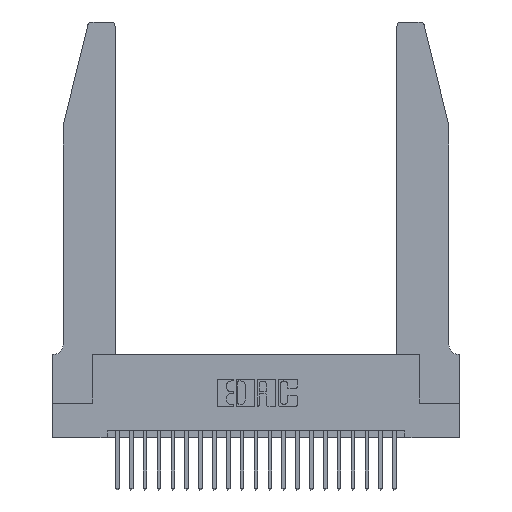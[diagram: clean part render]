
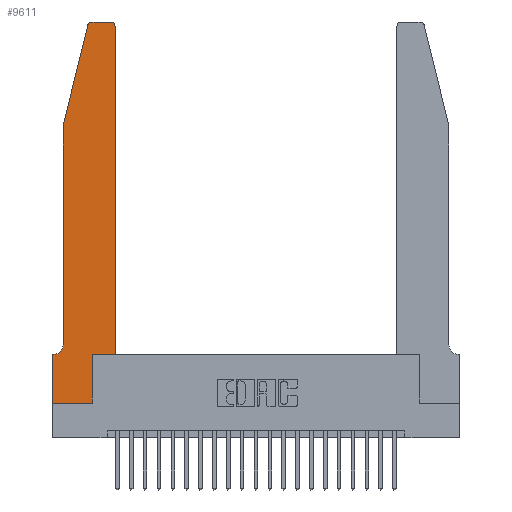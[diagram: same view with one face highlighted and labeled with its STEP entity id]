
A CAD part, top view. The second image highlights one B-rep face of the part: STEP entity #9611.
In plain terms, the highlighted planar face has unit normal (0, 0, 1).
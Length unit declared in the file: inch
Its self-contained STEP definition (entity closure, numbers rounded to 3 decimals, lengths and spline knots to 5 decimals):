
#337 = LINE ( 'NONE', #6783, #23899 ) ;
#454 = CARTESIAN_POINT ( 'NONE',  ( 0.4205, 2.75, 0.37 ) ) ;
#573 = CARTESIAN_POINT ( 'NONE',  ( 0.0055, 0.35, 0.37 ) ) ;
#661 = CARTESIAN_POINT ( 'NONE',  ( 0.284, 2.72, 0.37 ) ) ;
#675 = LINE ( 'NONE', #11678, #16179 ) ;
#829 = EDGE_CURVE ( 'NONE', #10533, #11977, #3335, .T. ) ;
#1005 = CARTESIAN_POINT ( 'NONE',  ( 0., 0.35, 0.37 ) ) ;
#1008 = EDGE_CURVE ( 'NONE', #17293, #2249, #337, .T. ) ;
#1236 = CARTESIAN_POINT ( 'NONE',  ( 0., 0., 0.37 ) ) ;
#1412 = ORIENTED_EDGE ( 'NONE', *, *, #17648, .T. ) ;
#1427 = AXIS2_PLACEMENT_3D ( 'NONE', #1005, #2926, #15957 ) ;
#1569 = AXIS2_PLACEMENT_3D ( 'NONE', #13085, #14661, #14747 ) ;
#1931 = ORIENTED_EDGE ( 'NONE', *, *, #8440, .T. ) ;
#2035 = VERTEX_POINT ( 'NONE', #454 ) ;
#2249 = VERTEX_POINT ( 'NONE', #2797 ) ;
#2597 = DIRECTION ( 'NONE',  ( 1., 0., 0. ) ) ;
#2797 = CARTESIAN_POINT ( 'NONE',  ( 0.4505, 0.35, 0.37 ) ) ;
#2926 = DIRECTION ( 'NONE',  ( 0., 0., 1. ) ) ;
#3052 = VECTOR ( 'NONE', #9074, 39.37008 ) ;
#3335 = CIRCLE ( 'NONE', #1569, 0.07 ) ;
#3887 = CARTESIAN_POINT ( 'NONE',  ( 0.4505, 2.72, 0.37 ) ) ;
#4028 = VECTOR ( 'NONE', #5595, 39.37008 ) ;
#4333 = CARTESIAN_POINT ( 'NONE',  ( 0.4205, 2.72, 0.37 ) ) ;
#5077 = VERTEX_POINT ( 'NONE', #14764 ) ;
#5273 = CARTESIAN_POINT ( 'NONE',  ( 0.0755, 2., 0.37 ) ) ;
#5348 = CARTESIAN_POINT ( 'NONE',  ( 0.2605, 2.75, 0.37 ) ) ;
#5595 = DIRECTION ( 'NONE',  ( -0.239, -0.971, 0. ) ) ;
#5989 = VECTOR ( 'NONE', #23496, 39.37008 ) ;
#6017 = CARTESIAN_POINT ( 'NONE',  ( 0.0755, 0.42, 0.37 ) ) ;
#6112 = ORIENTED_EDGE ( 'NONE', *, *, #19847, .T. ) ;
#6122 = CARTESIAN_POINT ( 'NONE',  ( 0.284, 2.75, 0.37 ) ) ;
#6222 = DIRECTION ( 'NONE',  ( 1., 0., 0. ) ) ;
#6243 = ORIENTED_EDGE ( 'NONE', *, *, #6863, .T. ) ;
#6483 = AXIS2_PLACEMENT_3D ( 'NONE', #4333, #17294, #6222 ) ;
#6542 = LINE ( 'NONE', #12704, #15240 ) ;
#6783 = CARTESIAN_POINT ( 'NONE',  ( 0.4505, 0.35, 0.37 ) ) ;
#6863 = EDGE_CURVE ( 'NONE', #7373, #2035, #22945, .T. ) ;
#7039 = EDGE_CURVE ( 'NONE', #11977, #12639, #9675, .T. ) ;
#7169 = CARTESIAN_POINT ( 'NONE',  ( 0.2865, 0.35, 0.37 ) ) ;
#7318 = CIRCLE ( 'NONE', #17016, 0.03 ) ;
#7373 = VERTEX_POINT ( 'NONE', #3887 ) ;
#7515 = ORIENTED_EDGE ( 'NONE', *, *, #11910, .T. ) ;
#7787 = VECTOR ( 'NONE', #13842, 39.37008 ) ;
#8080 = CARTESIAN_POINT ( 'NONE',  ( 0.2865, 0.35, 0.37 ) ) ;
#8278 = CARTESIAN_POINT ( 'NONE',  ( 0.4505, 0.35, 0.37 ) ) ;
#8440 = EDGE_CURVE ( 'NONE', #20515, #10632, #7318, .T. ) ;
#8659 = LINE ( 'NONE', #7169, #3052 ) ;
#8780 = ORIENTED_EDGE ( 'NONE', *, *, #829, .T. ) ;
#9074 = DIRECTION ( 'NONE',  ( 0., 1., 0. ) ) ;
#9082 = DIRECTION ( 'NONE',  ( 0., -1., 0. ) ) ;
#9112 = VECTOR ( 'NONE', #23492, 39.37008 ) ;
#9299 = EDGE_CURVE ( 'NONE', #10632, #19432, #18838, .T. ) ;
#9379 = EDGE_LOOP ( 'NONE', ( #1412, #1931, #19415, #7515, #8780, #14838, #13981, #6112, #17812, #16680, #15001, #6243 ) ) ;
#9611 = ADVANCED_FACE ( 'NONE', ( #16785 ), #12253, .T. ) ;
#9675 = LINE ( 'NONE', #14332, #9112 ) ;
#10533 = VERTEX_POINT ( 'NONE', #6017 ) ;
#10632 = VERTEX_POINT ( 'NONE', #11808 ) ;
#10966 = LINE ( 'NONE', #1236, #5989 ) ;
#11678 = CARTESIAN_POINT ( 'NONE',  ( 0.0755, 2., 0.37 ) ) ;
#11808 = CARTESIAN_POINT ( 'NONE',  ( 0.25487, 2.72718, 0.37 ) ) ;
#11910 = EDGE_CURVE ( 'NONE', #19432, #10533, #675, .T. ) ;
#11977 = VERTEX_POINT ( 'NONE', #573 ) ;
#12013 = EDGE_CURVE ( 'NONE', #2249, #7373, #22514, .T. ) ;
#12253 = PLANE ( 'NONE',  #1427 ) ;
#12639 = VERTEX_POINT ( 'NONE', #23385 ) ;
#12704 = CARTESIAN_POINT ( 'NONE',  ( 0., 0., 0.37 ) ) ;
#12822 = DIRECTION ( 'NONE',  ( -1., 0., 0. ) ) ;
#13085 = CARTESIAN_POINT ( 'NONE',  ( 0.0055, 0.42, 0.37 ) ) ;
#13764 = DIRECTION ( 'NONE',  ( 0., 0., 1. ) ) ;
#13842 = DIRECTION ( 'NONE',  ( 0., 1., 0. ) ) ;
#13981 = ORIENTED_EDGE ( 'NONE', *, *, #20868, .T. ) ;
#14332 = CARTESIAN_POINT ( 'NONE',  ( 0.0755, 0.35, 0.37 ) ) ;
#14661 = DIRECTION ( 'NONE',  ( 0., 0., -1. ) ) ;
#14747 = DIRECTION ( 'NONE',  ( -1., 0., 0. ) ) ;
#14764 = CARTESIAN_POINT ( 'NONE',  ( 0., 0., 0.37 ) ) ;
#14838 = ORIENTED_EDGE ( 'NONE', *, *, #7039, .T. ) ;
#15001 = ORIENTED_EDGE ( 'NONE', *, *, #12013, .T. ) ;
#15240 = VECTOR ( 'NONE', #9082, 39.37008 ) ;
#15957 = DIRECTION ( 'NONE',  ( 1., 0., 0. ) ) ;
#16179 = VECTOR ( 'NONE', #22716, 39.37008 ) ;
#16632 = DIRECTION ( 'NONE',  ( 1., 0., 0. ) ) ;
#16680 = ORIENTED_EDGE ( 'NONE', *, *, #1008, .T. ) ;
#16785 = FACE_OUTER_BOUND ( 'NONE', #9379, .T. ) ;
#17016 = AXIS2_PLACEMENT_3D ( 'NONE', #661, #13764, #2597 ) ;
#17048 = VECTOR ( 'NONE', #12822, 39.37008 ) ;
#17293 = VERTEX_POINT ( 'NONE', #8080 ) ;
#17294 = DIRECTION ( 'NONE',  ( 0., 0., 1. ) ) ;
#17648 = EDGE_CURVE ( 'NONE', #2035, #20515, #21978, .T. ) ;
#17812 = ORIENTED_EDGE ( 'NONE', *, *, #18822, .T. ) ;
#18822 = EDGE_CURVE ( 'NONE', #20705, #17293, #8659, .T. ) ;
#18838 = LINE ( 'NONE', #20520, #4028 ) ;
#19415 = ORIENTED_EDGE ( 'NONE', *, *, #9299, .T. ) ;
#19432 = VERTEX_POINT ( 'NONE', #5273 ) ;
#19651 = CARTESIAN_POINT ( 'NONE',  ( 0.2865, 0., 0.37 ) ) ;
#19847 = EDGE_CURVE ( 'NONE', #5077, #20705, #10966, .T. ) ;
#20515 = VERTEX_POINT ( 'NONE', #6122 ) ;
#20520 = CARTESIAN_POINT ( 'NONE',  ( 0.0755, 2., 0.37 ) ) ;
#20705 = VERTEX_POINT ( 'NONE', #19651 ) ;
#20868 = EDGE_CURVE ( 'NONE', #12639, #5077, #6542, .T. ) ;
#21978 = LINE ( 'NONE', #5348, #17048 ) ;
#22514 = LINE ( 'NONE', #8278, #7787 ) ;
#22716 = DIRECTION ( 'NONE',  ( 0., -1., 0. ) ) ;
#22945 = CIRCLE ( 'NONE', #6483, 0.03 ) ;
#23385 = CARTESIAN_POINT ( 'NONE',  ( 0., 0.35, 0.37 ) ) ;
#23492 = DIRECTION ( 'NONE',  ( -1., 0., 0. ) ) ;
#23496 = DIRECTION ( 'NONE',  ( 1., 0., 0. ) ) ;
#23899 = VECTOR ( 'NONE', #16632, 39.37008 ) ;
